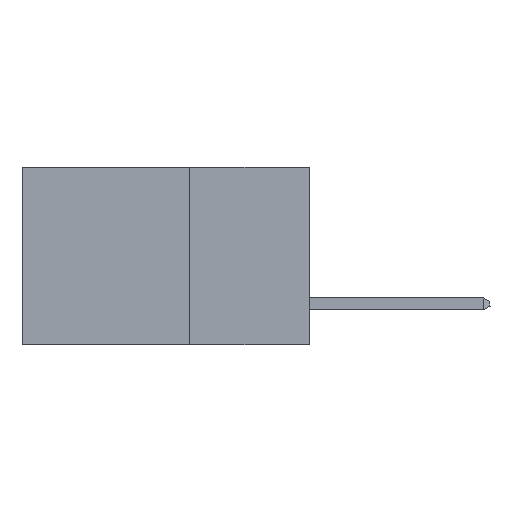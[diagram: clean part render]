
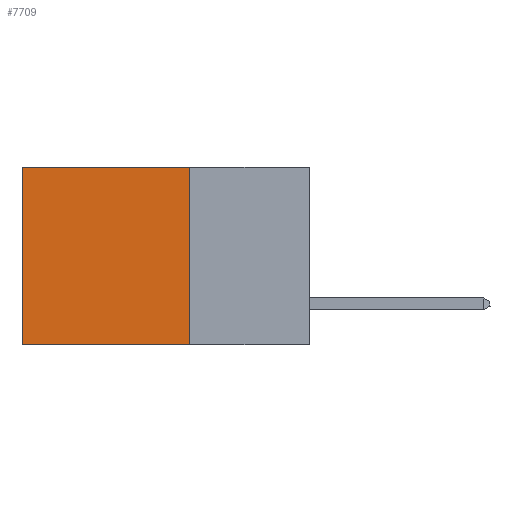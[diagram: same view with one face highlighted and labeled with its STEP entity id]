
A CAD part, left-side view. The second image highlights one B-rep face of the part: STEP entity #7709.
In plain terms, the highlighted planar face has unit normal (-1, 0, 0).
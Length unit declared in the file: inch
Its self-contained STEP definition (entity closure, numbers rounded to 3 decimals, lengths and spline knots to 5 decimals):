
#189 = LINE ( 'NONE', #3580, #20108 ) ;
#754 = DIRECTION ( 'NONE',  ( 0., 1., 0. ) ) ;
#838 = DIRECTION ( 'NONE',  ( 0., 0., -1. ) ) ;
#1442 = VECTOR ( 'NONE', #14202, 39.37008 ) ;
#2054 = ORIENTED_EDGE ( 'NONE', *, *, #22381, .T. ) ;
#2127 = VECTOR ( 'NONE', #18577, 39.37008 ) ;
#3580 = CARTESIAN_POINT ( 'NONE',  ( 0.2875, 0.25, 0. ) ) ;
#3653 = DIRECTION ( 'NONE',  ( 0., 1., 0. ) ) ;
#3707 = VERTEX_POINT ( 'NONE', #22094 ) ;
#6741 = VERTEX_POINT ( 'NONE', #15831 ) ;
#7190 = CARTESIAN_POINT ( 'NONE',  ( 0.2875, 0.25, -0.37 ) ) ;
#7709 = ADVANCED_FACE ( 'NONE', ( #8603 ), #21618, .F. ) ;
#7862 = CARTESIAN_POINT ( 'NONE',  ( 0.2875, 0.6, 0. ) ) ;
#8551 = EDGE_LOOP ( 'NONE', ( #2054, #13159, #14705, #14768 ) ) ;
#8603 = FACE_OUTER_BOUND ( 'NONE', #8551, .T. ) ;
#9128 = LINE ( 'NONE', #7190, #17113 ) ;
#9200 = CARTESIAN_POINT ( 'NONE',  ( 0.2875, 0.25, 0. ) ) ;
#9736 = DIRECTION ( 'NONE',  ( 1., 0., 0. ) ) ;
#11150 = EDGE_CURVE ( 'NONE', #6741, #14314, #189, .T. ) ;
#13159 = ORIENTED_EDGE ( 'NONE', *, *, #21639, .F. ) ;
#13500 = LINE ( 'NONE', #7862, #2127 ) ;
#13745 = VERTEX_POINT ( 'NONE', #15209 ) ;
#14202 = DIRECTION ( 'NONE',  ( 0., 0., -1. ) ) ;
#14309 = CARTESIAN_POINT ( 'NONE',  ( 0.2875, 0.6, 0. ) ) ;
#14314 = VERTEX_POINT ( 'NONE', #14309 ) ;
#14500 = LINE ( 'NONE', #9200, #1442 ) ;
#14705 = ORIENTED_EDGE ( 'NONE', *, *, #19091, .F. ) ;
#14768 = ORIENTED_EDGE ( 'NONE', *, *, #11150, .T. ) ;
#15209 = CARTESIAN_POINT ( 'NONE',  ( 0.2875, 0.6, -0.37 ) ) ;
#15831 = CARTESIAN_POINT ( 'NONE',  ( 0.2875, 0.25, 0. ) ) ;
#17113 = VECTOR ( 'NONE', #754, 39.37008 ) ;
#18577 = DIRECTION ( 'NONE',  ( 0., 0., -1. ) ) ;
#19091 = EDGE_CURVE ( 'NONE', #6741, #3707, #14500, .T. ) ;
#19594 = AXIS2_PLACEMENT_3D ( 'NONE', #22152, #9736, #838 ) ;
#20108 = VECTOR ( 'NONE', #3653, 39.37008 ) ;
#21618 = PLANE ( 'NONE',  #19594 ) ;
#21639 = EDGE_CURVE ( 'NONE', #3707, #13745, #9128, .T. ) ;
#22094 = CARTESIAN_POINT ( 'NONE',  ( 0.2875, 0.25, -0.37 ) ) ;
#22152 = CARTESIAN_POINT ( 'NONE',  ( 0.2875, 0.25, 0. ) ) ;
#22381 = EDGE_CURVE ( 'NONE', #14314, #13745, #13500, .T. ) ;
